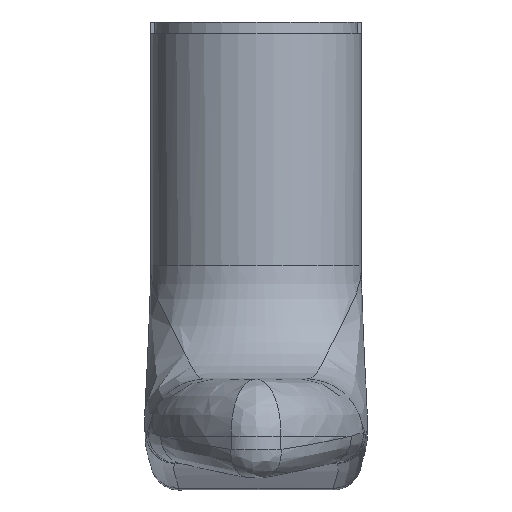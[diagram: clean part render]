
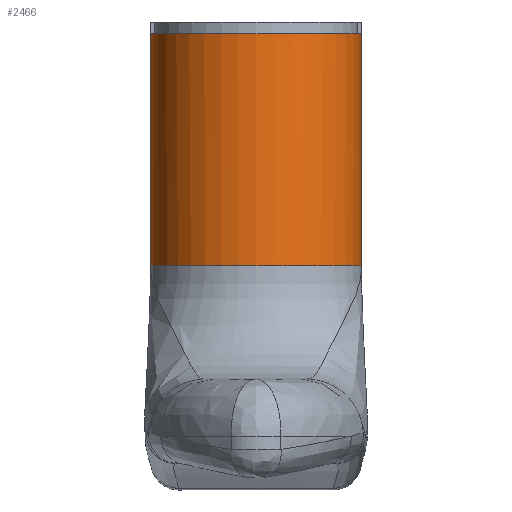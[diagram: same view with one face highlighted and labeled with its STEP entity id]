
A CAD part, front view. The second image highlights one B-rep face of the part: STEP entity #2466.
In plain terms, the highlighted cylindrical face has radius 18.575 mm (diameter 37.15 mm), a partial arc.
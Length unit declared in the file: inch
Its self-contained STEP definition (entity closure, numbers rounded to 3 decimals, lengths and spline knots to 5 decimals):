
#93 = AXIS2_PLACEMENT_3D ( 'NONE', #772, #2569, #1035 ) ;
#122 = CARTESIAN_POINT ( 'NONE',  ( 0.0002, 1.90601, -9.97725 ) ) ;
#167 = VECTOR ( 'NONE', #2105, 39.37008 ) ;
#200 = CARTESIAN_POINT ( 'NONE',  ( 1.4603, 1.88022, -9.9334 ) ) ;
#227 = CARTESIAN_POINT ( 'NONE',  ( 1.4603, 1.88022, -9.9334 ) ) ;
#233 = VERTEX_POINT ( 'NONE', #2012 ) ;
#242 = CARTESIAN_POINT ( 'NONE',  ( 1.46171, 1.90529, -9.97483 ) ) ;
#295 = ORIENTED_EDGE ( 'NONE', *, *, #794, .T. ) ;
#385 = CARTESIAN_POINT ( 'NONE',  ( 0.00021, 1.90569, -9.97615 ) ) ;
#397 = CARTESIAN_POINT ( 'NONE',  ( 0.73097, 1.93382, -2.18005 ) ) ;
#446 = FACE_OUTER_BOUND ( 'NONE', #2875, .T. ) ;
#507 = CARTESIAN_POINT ( 'NONE',  ( 1.46177, 1.90674, -9.97965 ) ) ;
#641 = CARTESIAN_POINT ( 'NONE',  ( 0.00026, 1.90431, -9.97157 ) ) ;
#705 = VECTOR ( 'NONE', #1226, 39.37008 ) ;
#737 = CARTESIAN_POINT ( 'NONE',  ( 1.46072, 1.88618, -9.93958 ) ) ;
#749 = CARTESIAN_POINT ( 'NONE',  ( 1.46184, 1.90894, -9.98965 ) ) ;
#772 = CARTESIAN_POINT ( 'NONE',  ( 0.73097, 1.93382, -8.32484 ) ) ;
#794 = EDGE_CURVE ( 'NONE', #1182, #1461, #808, .T. ) ;
#808 = LINE ( 'NONE', #1484, #705 ) ;
#823 = ORIENTED_EDGE ( 'NONE', *, *, #2433, .T. ) ;
#890 = CARTESIAN_POINT ( 'NONE',  ( 0.00047, 1.89959, -9.96001 ) ) ;
#935 = VERTEX_POINT ( 'NONE', #2786 ) ;
#979 = CARTESIAN_POINT ( 'NONE',  ( 0., 1.91183, -8.32484 ) ) ;
#995 = CIRCLE ( 'NONE', #93, 0.7313 ) ;
#996 = CARTESIAN_POINT ( 'NONE',  ( 1.46117, 1.89372, -9.94956 ) ) ;
#1012 = CARTESIAN_POINT ( 'NONE',  ( 1.46188, 1.91004, -9.99645 ) ) ;
#1016 = CARTESIAN_POINT ( 'NONE',  ( 0.73097, 1.93382, -9.9334 ) ) ;
#1035 = DIRECTION ( 'NONE',  ( 1., 0., 0. ) ) ;
#1131 = AXIS2_PLACEMENT_3D ( 'NONE', #397, #1925, #2447 ) ;
#1140 = CARTESIAN_POINT ( 'NONE',  ( 0.00002, 1.91131, -10.00668 ) ) ;
#1148 = CARTESIAN_POINT ( 'NONE',  ( 0.00088, 1.89159, -9.94596 ) ) ;
#1182 = VERTEX_POINT ( 'NONE', #979 ) ;
#1188 = EDGE_CURVE ( 'NONE', #2952, #935, #1455, .T. ) ;
#1226 = DIRECTION ( 'NONE',  ( 0., 0., -1. ) ) ;
#1257 = CARTESIAN_POINT ( 'NONE',  ( 1.46147, 1.89963, -9.96009 ) ) ;
#1272 = CARTESIAN_POINT ( 'NONE',  ( 1.46189, 1.91039, -9.99913 ) ) ;
#1275 = DIRECTION ( 'NONE',  ( 1., 0., 0. ) ) ;
#1327 = CARTESIAN_POINT ( 'NONE',  ( 0.00164, 1.88022, -9.9334 ) ) ;
#1349 = VERTEX_POINT ( 'NONE', #1327 ) ;
#1395 = CARTESIAN_POINT ( 'NONE',  ( 0.0001, 1.90876, -9.98843 ) ) ;
#1407 = CARTESIAN_POINT ( 'NONE',  ( 0.00164, 1.88022, -9.9334 ) ) ;
#1455 = B_SPLINE_CURVE_WITH_KNOTS ( 'NONE', 3,
 ( #227, #2265, #737, #2533, #996, #2783, #1257, #3042, #1514, #3297, #1777, #242, #2024, #507, #2282, #749, #2548, #1012, #2799, #1272, #3057, #1530, #3310, #1793 ),
 .UNSPECIFIED., .F., .F.,
 ( 4, 2, 2, 2, 1, 1, 2, 2, 2, 1, 1, 2, 2, 4 ),
 ( 0., 0.125, 0.25, 0.375, 0.4375, 0.46875, 0.48438, 0.5, 0.625, 0.6875, 0.71875, 0.73438, 0.75, 1. ),
 .UNSPECIFIED. ) ;
#1461 = VERTEX_POINT ( 'NONE', #2816 ) ;
#1484 = CARTESIAN_POINT ( 'NONE',  ( 0., 1.91183, -2.18005 ) ) ;
#1514 = CARTESIAN_POINT ( 'NONE',  ( 1.46163, 1.90325, -9.96873 ) ) ;
#1522 = LINE ( 'NONE', #2822, #167 ) ;
#1530 = CARTESIAN_POINT ( 'NONE',  ( 1.46192, 1.91139, -10.0077 ) ) ;
#1591 = ORIENTED_EDGE ( 'NONE', *, *, #2473, .T. ) ;
#1654 = CARTESIAN_POINT ( 'NONE',  ( 0.00018, 1.90645, -9.97879 ) ) ;
#1716 = CYLINDRICAL_SURFACE ( 'NONE', #1131, 0.7313 ) ;
#1777 = CARTESIAN_POINT ( 'NONE',  ( 1.4617, 1.90497, -9.9738 ) ) ;
#1785 = CARTESIAN_POINT ( 'NONE',  ( 0., 1.91183, -10.02504 ) ) ;
#1793 = CARTESIAN_POINT ( 'NONE',  ( 1.46194, 1.91183, -10.02504 ) ) ;
#1864 = ORIENTED_EDGE ( 'NONE', *, *, #1188, .T. ) ;
#1907 = CARTESIAN_POINT ( 'NONE',  ( 0.00021, 1.90582, -9.97659 ) ) ;
#1922 = EDGE_CURVE ( 'NONE', #1182, #233, #995, .T. ) ;
#1925 = DIRECTION ( 'NONE',  ( 0., 0., -1. ) ) ;
#1966 = EDGE_CURVE ( 'NONE', #233, #935, #1522, .T. ) ;
#1994 = AXIS2_PLACEMENT_3D ( 'NONE', #1016, #2802, #1275 ) ;
#2012 = CARTESIAN_POINT ( 'NONE',  ( 1.46194, 1.91183, -8.32484 ) ) ;
#2024 = CARTESIAN_POINT ( 'NONE',  ( 1.46172, 1.90546, -9.9754 ) ) ;
#2032 = CARTESIAN_POINT ( 'NONE',  ( 0., 1.91183, -10.01554 ) ) ;
#2094 = ORIENTED_EDGE ( 'NONE', *, *, #1922, .F. ) ;
#2105 = DIRECTION ( 'NONE',  ( 0., 0., -1. ) ) ;
#2166 = CARTESIAN_POINT ( 'NONE',  ( 0.00021, 1.90564, -9.97598 ) ) ;
#2265 = CARTESIAN_POINT ( 'NONE',  ( 1.46053, 1.88333, -9.93643 ) ) ;
#2279 = ORIENTED_EDGE ( 'NONE', *, *, #1966, .F. ) ;
#2282 = CARTESIAN_POINT ( 'NONE',  ( 1.4618, 1.90771, -9.98357 ) ) ;
#2339 = B_SPLINE_CURVE_WITH_KNOTS ( 'NONE', 3,
 ( #1785, #2032, #1140, #2933, #1395, #3185, #1654, #122, #1907, #385, #2166, #641, #2427, #890, #2678, #1148, #2941, #1407 ),
 .UNSPECIFIED., .F., .F.,
 ( 4, 2, 1, 1, 1, 1, 2, 2, 2, 2, 4 ),
 ( 0., 0.25, 0.375, 0.4375, 0.46875, 0.48437, 0.49219, 0.5, 0.625, 0.75, 1. ),
 .UNSPECIFIED. ) ;
#2421 = CIRCLE ( 'NONE', #1994, 0.7313 ) ;
#2427 = CARTESIAN_POINT ( 'NONE',  ( 0.00032, 1.90287, -9.9676 ) ) ;
#2433 = EDGE_CURVE ( 'NONE', #1461, #1349, #2339, .T. ) ;
#2447 = DIRECTION ( 'NONE',  ( -1., 0., 0. ) ) ;
#2466 = ADVANCED_FACE ( 'NONE', ( #446 ), #1716, .T. ) ;
#2473 = EDGE_CURVE ( 'NONE', #1349, #2952, #2421, .T. ) ;
#2533 = CARTESIAN_POINT ( 'NONE',  ( 1.46104, 1.89136, -9.94611 ) ) ;
#2548 = CARTESIAN_POINT ( 'NONE',  ( 1.46186, 1.9095, -9.99275 ) ) ;
#2569 = DIRECTION ( 'NONE',  ( 0., 0., 1. ) ) ;
#2678 = CARTESIAN_POINT ( 'NONE',  ( 0.00055, 1.89779, -9.95645 ) ) ;
#2783 = CARTESIAN_POINT ( 'NONE',  ( 1.46138, 1.89779, -9.95646 ) ) ;
#2786 = CARTESIAN_POINT ( 'NONE',  ( 1.46194, 1.91183, -10.02504 ) ) ;
#2799 = CARTESIAN_POINT ( 'NONE',  ( 1.46189, 1.91025, -9.99805 ) ) ;
#2802 = DIRECTION ( 'NONE',  ( 0., 0., 1. ) ) ;
#2816 = CARTESIAN_POINT ( 'NONE',  ( 0., 1.91183, -10.02504 ) ) ;
#2822 = CARTESIAN_POINT ( 'NONE',  ( 1.46194, 1.91183, -2.18005 ) ) ;
#2875 = EDGE_LOOP ( 'NONE', ( #2279, #2094, #295, #823, #1591, #1864 ) ) ;
#2933 = CARTESIAN_POINT ( 'NONE',  ( 0.00007, 1.90974, -9.99435 ) ) ;
#2941 = CARTESIAN_POINT ( 'NONE',  ( 0.00118, 1.88642, -9.93944 ) ) ;
#2952 = VERTEX_POINT ( 'NONE', #200 ) ;
#3042 = CARTESIAN_POINT ( 'NONE',  ( 1.46158, 1.90209, -9.9658 ) ) ;
#3057 = CARTESIAN_POINT ( 'NONE',  ( 1.46189, 1.91046, -9.99974 ) ) ;
#3185 = CARTESIAN_POINT ( 'NONE',  ( 0.00015, 1.90727, -9.98193 ) ) ;
#3297 = CARTESIAN_POINT ( 'NONE',  ( 1.46168, 1.90447, -9.97226 ) ) ;
#3310 = CARTESIAN_POINT ( 'NONE',  ( 1.46194, 1.91183, -10.01598 ) ) ;
